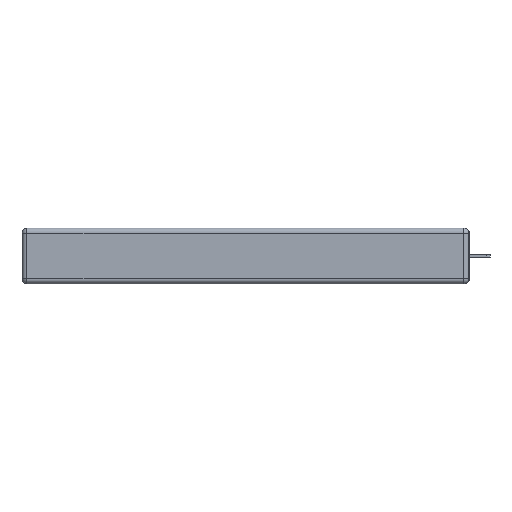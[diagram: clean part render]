
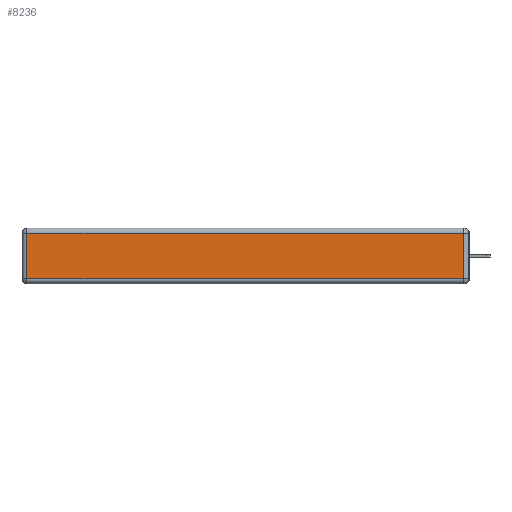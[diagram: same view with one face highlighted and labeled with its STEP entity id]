
A CAD part, left-side view. The second image highlights one B-rep face of the part: STEP entity #8236.
In plain terms, the highlighted planar face has unit normal (-1, 0, 0).
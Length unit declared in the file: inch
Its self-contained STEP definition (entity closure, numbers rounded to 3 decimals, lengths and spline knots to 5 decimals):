
#875 = DIRECTION ( 'NONE',  ( 0., -1., 0. ) ) ;
#2038 = CARTESIAN_POINT ( 'NONE',  ( 0., 2.75, -0.03 ) ) ;
#2876 = CARTESIAN_POINT ( 'NONE',  ( 0., 0.03, -0.313 ) ) ;
#3092 = DIRECTION ( 'NONE',  ( 0., 0., -1. ) ) ;
#3112 = VERTEX_POINT ( 'NONE', #2876 ) ;
#3469 = ORIENTED_EDGE ( 'NONE', *, *, #6067, .T. ) ;
#5047 = CARTESIAN_POINT ( 'NONE',  ( 0., 0.03, -0.03 ) ) ;
#5100 = DIRECTION ( 'NONE',  ( -1., 0., 0. ) ) ;
#5789 = CARTESIAN_POINT ( 'NONE',  ( 0., 2.72, -0.03 ) ) ;
#5997 = FACE_OUTER_BOUND ( 'NONE', #8989, .T. ) ;
#6067 = EDGE_CURVE ( 'NONE', #6822, #3112, #8503, .T. ) ;
#6237 = EDGE_CURVE ( 'NONE', #3112, #10951, #7977, .T. ) ;
#6783 = VECTOR ( 'NONE', #3092, 39.37008 ) ;
#6822 = VERTEX_POINT ( 'NONE', #12745 ) ;
#7741 = VECTOR ( 'NONE', #875, 39.37008 ) ;
#7977 = LINE ( 'NONE', #13597, #14331 ) ;
#8236 = ADVANCED_FACE ( 'NONE', ( #5997 ), #9625, .T. ) ;
#8503 = LINE ( 'NONE', #14110, #7741 ) ;
#8504 = CARTESIAN_POINT ( 'NONE',  ( 0., 2.72, -0.343 ) ) ;
#8989 = EDGE_LOOP ( 'NONE', ( #3469, #13527, #12848, #9081 ) ) ;
#9081 = ORIENTED_EDGE ( 'NONE', *, *, #12461, .T. ) ;
#9161 = DIRECTION ( 'NONE',  ( 0., 0., 1. ) ) ;
#9323 = CARTESIAN_POINT ( 'NONE',  ( 0., 0., -0.343 ) ) ;
#9389 = VERTEX_POINT ( 'NONE', #5789 ) ;
#9625 = PLANE ( 'NONE',  #14132 ) ;
#9770 = LINE ( 'NONE', #2038, #11055 ) ;
#10570 = DIRECTION ( 'NONE',  ( 0., 0., 1. ) ) ;
#10951 = VERTEX_POINT ( 'NONE', #5047 ) ;
#10997 = LINE ( 'NONE', #8504, #6783 ) ;
#11055 = VECTOR ( 'NONE', #14257, 39.37008 ) ;
#12461 = EDGE_CURVE ( 'NONE', #9389, #6822, #10997, .T. ) ;
#12745 = CARTESIAN_POINT ( 'NONE',  ( 0., 2.72, -0.313 ) ) ;
#12848 = ORIENTED_EDGE ( 'NONE', *, *, #13616, .T. ) ;
#13527 = ORIENTED_EDGE ( 'NONE', *, *, #6237, .T. ) ;
#13597 = CARTESIAN_POINT ( 'NONE',  ( 0., 0.03, -0.343 ) ) ;
#13616 = EDGE_CURVE ( 'NONE', #10951, #9389, #9770, .T. ) ;
#14110 = CARTESIAN_POINT ( 'NONE',  ( 0., 0., -0.313 ) ) ;
#14132 = AXIS2_PLACEMENT_3D ( 'NONE', #9323, #5100, #10570 ) ;
#14257 = DIRECTION ( 'NONE',  ( 0., 1., 0. ) ) ;
#14331 = VECTOR ( 'NONE', #9161, 39.37008 ) ;
